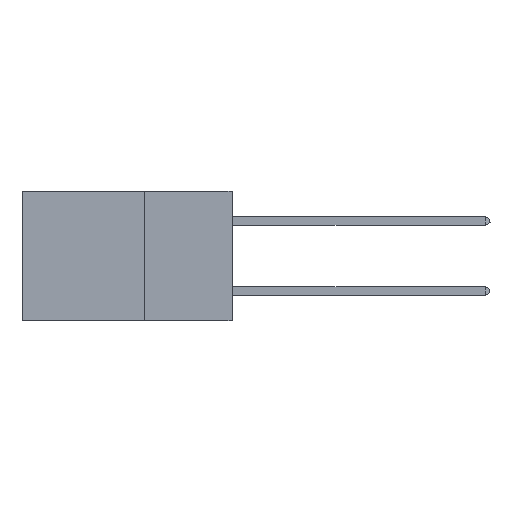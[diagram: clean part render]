
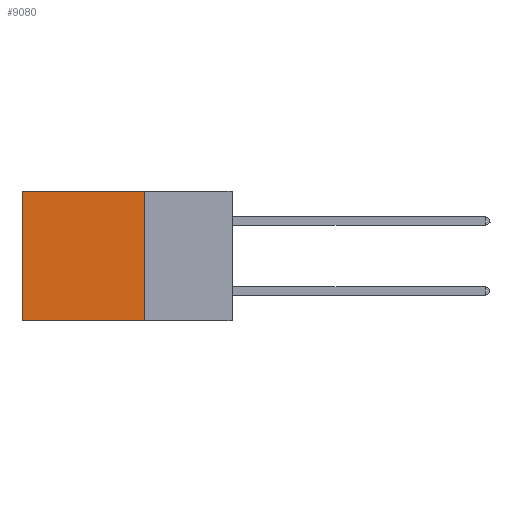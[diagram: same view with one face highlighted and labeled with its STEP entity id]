
A CAD part, left-side view. The second image highlights one B-rep face of the part: STEP entity #9080.
In plain terms, the highlighted planar face has unit normal (-1, 0, 0).
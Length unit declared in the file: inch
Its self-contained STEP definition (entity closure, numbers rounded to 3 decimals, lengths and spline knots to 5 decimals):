
#701 = DIRECTION ( 'NONE',  ( 0., 0., -1. ) ) ;
#1299 = EDGE_CURVE ( 'NONE', #19285, #18484, #11010, .T. ) ;
#1626 = EDGE_CURVE ( 'NONE', #18484, #8383, #8208, .T. ) ;
#1989 = DIRECTION ( 'NONE',  ( 1., 0., 0. ) ) ;
#2822 = VECTOR ( 'NONE', #9650, 39.37008 ) ;
#3770 = CARTESIAN_POINT ( 'NONE',  ( 0.2875, 0.25, -0.37 ) ) ;
#3971 = CARTESIAN_POINT ( 'NONE',  ( 0.2875, 0.25, 0. ) ) ;
#5043 = AXIS2_PLACEMENT_3D ( 'NONE', #3971, #1989, #15915 ) ;
#8208 = LINE ( 'NONE', #23247, #2822 ) ;
#8383 = VERTEX_POINT ( 'NONE', #25099 ) ;
#8511 = LINE ( 'NONE', #25190, #13736 ) ;
#9080 = ADVANCED_FACE ( 'NONE', ( #12585 ), #13948, .F. ) ;
#9223 = CARTESIAN_POINT ( 'NONE',  ( 0.2875, 0.25, 0. ) ) ;
#9650 = DIRECTION ( 'NONE',  ( 0., 0., -1. ) ) ;
#9885 = LINE ( 'NONE', #24390, #24726 ) ;
#10386 = VECTOR ( 'NONE', #20482, 39.37008 ) ;
#11010 = LINE ( 'NONE', #18444, #10386 ) ;
#11699 = DIRECTION ( 'NONE',  ( 0., 1., 0. ) ) ;
#11917 = ORIENTED_EDGE ( 'NONE', *, *, #17339, .F. ) ;
#12514 = EDGE_LOOP ( 'NONE', ( #24551, #13700, #11917, #24640 ) ) ;
#12585 = FACE_OUTER_BOUND ( 'NONE', #12514, .T. ) ;
#12708 = CARTESIAN_POINT ( 'NONE',  ( 0.2875, 0.6, 0. ) ) ;
#13700 = ORIENTED_EDGE ( 'NONE', *, *, #16306, .F. ) ;
#13736 = VECTOR ( 'NONE', #11699, 39.37008 ) ;
#13948 = PLANE ( 'NONE',  #5043 ) ;
#15915 = DIRECTION ( 'NONE',  ( 0., 0., -1. ) ) ;
#16306 = EDGE_CURVE ( 'NONE', #23544, #8383, #8511, .T. ) ;
#17339 = EDGE_CURVE ( 'NONE', #19285, #23544, #9885, .T. ) ;
#18444 = CARTESIAN_POINT ( 'NONE',  ( 0.2875, 0.25, 0. ) ) ;
#18484 = VERTEX_POINT ( 'NONE', #12708 ) ;
#19285 = VERTEX_POINT ( 'NONE', #9223 ) ;
#20482 = DIRECTION ( 'NONE',  ( 0., 1., 0. ) ) ;
#23247 = CARTESIAN_POINT ( 'NONE',  ( 0.2875, 0.6, 0. ) ) ;
#23544 = VERTEX_POINT ( 'NONE', #3770 ) ;
#24390 = CARTESIAN_POINT ( 'NONE',  ( 0.2875, 0.25, 0. ) ) ;
#24551 = ORIENTED_EDGE ( 'NONE', *, *, #1626, .T. ) ;
#24640 = ORIENTED_EDGE ( 'NONE', *, *, #1299, .T. ) ;
#24726 = VECTOR ( 'NONE', #701, 39.37008 ) ;
#25099 = CARTESIAN_POINT ( 'NONE',  ( 0.2875, 0.6, -0.37 ) ) ;
#25190 = CARTESIAN_POINT ( 'NONE',  ( 0.2875, 0.25, -0.37 ) ) ;
